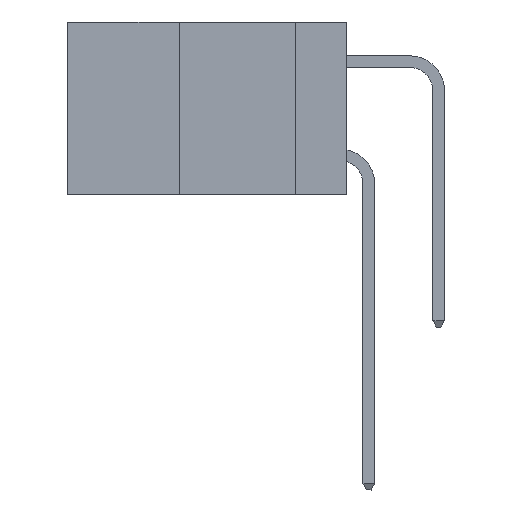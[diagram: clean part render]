
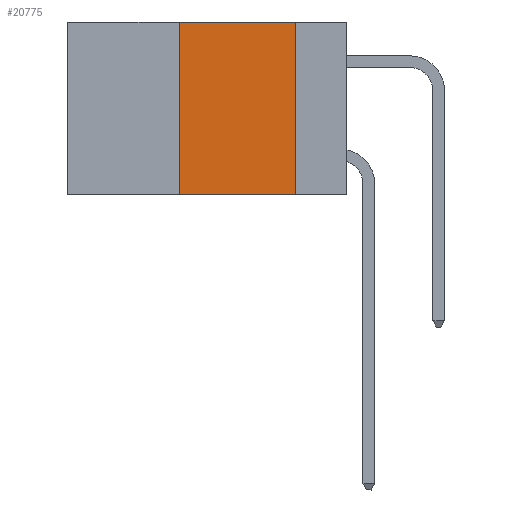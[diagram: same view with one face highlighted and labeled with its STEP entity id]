
A CAD part, left-side view. The second image highlights one B-rep face of the part: STEP entity #20775.
In plain terms, the highlighted planar face has unit normal (-1, 0, 0).
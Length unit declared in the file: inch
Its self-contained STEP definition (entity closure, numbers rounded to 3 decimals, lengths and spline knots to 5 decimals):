
#73 = CARTESIAN_POINT ( 'NONE',  ( 0., 0.11, 0. ) ) ;
#139 = VECTOR ( 'NONE', #8577, 39.37008 ) ;
#947 = LINE ( 'NONE', #12379, #16604 ) ;
#1352 = EDGE_CURVE ( 'NONE', #6961, #4846, #18234, .T. ) ;
#1782 = ORIENTED_EDGE ( 'NONE', *, *, #20119, .F. ) ;
#2378 = DIRECTION ( 'NONE',  ( 0., 0., -1. ) ) ;
#3709 = ORIENTED_EDGE ( 'NONE', *, *, #6723, .T. ) ;
#4846 = VERTEX_POINT ( 'NONE', #19597 ) ;
#5958 = VECTOR ( 'NONE', #12586, 39.37008 ) ;
#6723 = EDGE_CURVE ( 'NONE', #6961, #7939, #947, .T. ) ;
#6944 = LINE ( 'NONE', #18554, #11737 ) ;
#6961 = VERTEX_POINT ( 'NONE', #16481 ) ;
#7939 = VERTEX_POINT ( 'NONE', #11579 ) ;
#8577 = DIRECTION ( 'NONE',  ( 0., -1., 0. ) ) ;
#9303 = CARTESIAN_POINT ( 'NONE',  ( 0., 0.36, 0. ) ) ;
#10909 = DIRECTION ( 'NONE',  ( 1., 0., 0. ) ) ;
#11012 = DIRECTION ( 'NONE',  ( 0., 0., -1. ) ) ;
#11014 = EDGE_CURVE ( 'NONE', #4846, #20005, #17875, .T. ) ;
#11579 = CARTESIAN_POINT ( 'NONE',  ( 0., 0.11, -0.37 ) ) ;
#11737 = VECTOR ( 'NONE', #2378, 39.37008 ) ;
#11869 = CARTESIAN_POINT ( 'NONE',  ( 0., 0.6, 0. ) ) ;
#12379 = CARTESIAN_POINT ( 'NONE',  ( 0., 0.6, -0.37 ) ) ;
#12586 = DIRECTION ( 'NONE',  ( 0., 0., 1. ) ) ;
#14189 = FACE_OUTER_BOUND ( 'NONE', #19797, .T. ) ;
#16481 = CARTESIAN_POINT ( 'NONE',  ( 0., 0.36, -0.37 ) ) ;
#16604 = VECTOR ( 'NONE', #19993, 39.37008 ) ;
#17429 = ORIENTED_EDGE ( 'NONE', *, *, #11014, .F. ) ;
#17875 = LINE ( 'NONE', #11869, #139 ) ;
#18234 = LINE ( 'NONE', #9303, #5958 ) ;
#18554 = CARTESIAN_POINT ( 'NONE',  ( 0., 0.11, 0. ) ) ;
#18824 = AXIS2_PLACEMENT_3D ( 'NONE', #20641, #10909, #11012 ) ;
#19386 = ORIENTED_EDGE ( 'NONE', *, *, #1352, .F. ) ;
#19597 = CARTESIAN_POINT ( 'NONE',  ( 0., 0.36, 0. ) ) ;
#19797 = EDGE_LOOP ( 'NONE', ( #1782, #17429, #19386, #3709 ) ) ;
#19993 = DIRECTION ( 'NONE',  ( 0., -1., 0. ) ) ;
#20005 = VERTEX_POINT ( 'NONE', #73 ) ;
#20119 = EDGE_CURVE ( 'NONE', #20005, #7939, #6944, .T. ) ;
#20214 = PLANE ( 'NONE',  #18824 ) ;
#20641 = CARTESIAN_POINT ( 'NONE',  ( 0., 0.6, 0. ) ) ;
#20775 = ADVANCED_FACE ( 'NONE', ( #14189 ), #20214, .F. ) ;
